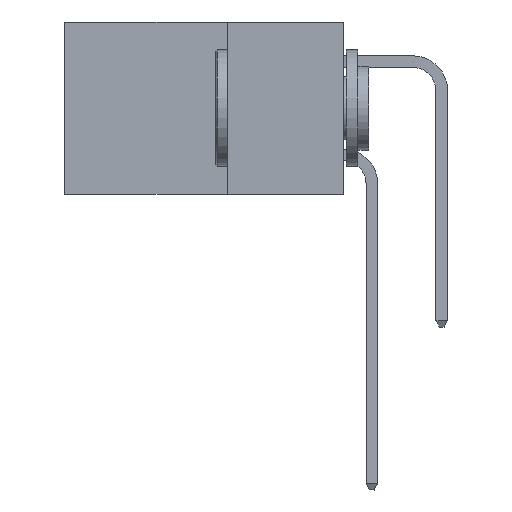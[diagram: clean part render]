
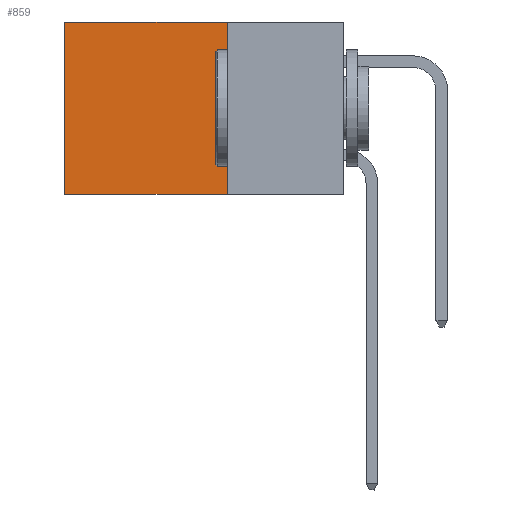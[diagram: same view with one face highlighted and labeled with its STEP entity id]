
A CAD part, left-side view. The second image highlights one B-rep face of the part: STEP entity #859.
In plain terms, the highlighted planar face has unit normal (-1, 0, 0).
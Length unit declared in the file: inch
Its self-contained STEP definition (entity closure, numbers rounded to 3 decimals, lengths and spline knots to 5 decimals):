
#859 = ADVANCED_FACE ( 'NONE', ( #1361 ), #1372, .F. ) ;
#956 = EDGE_CURVE ( 'NONE', #3235, #8880, #4372, .T. ) ;
#1049 = VECTOR ( 'NONE', #12435, 39.37008 ) ;
#1361 = FACE_OUTER_BOUND ( 'NONE', #3888, .T. ) ;
#1372 = PLANE ( 'NONE',  #4037 ) ;
#1467 = CARTESIAN_POINT ( 'NONE',  ( 0.298, 0.6, 0. ) ) ;
#2017 = VECTOR ( 'NONE', #2345, 39.37008 ) ;
#2297 = EDGE_CURVE ( 'NONE', #3453, #7307, #4333, .T. ) ;
#2336 = ORIENTED_EDGE ( 'NONE', *, *, #2297, .T. ) ;
#2345 = DIRECTION ( 'NONE',  ( 0., 1., 0. ) ) ;
#3235 = VERTEX_POINT ( 'NONE', #12936 ) ;
#3274 = DIRECTION ( 'NONE',  ( 0., 0., -1. ) ) ;
#3366 = DIRECTION ( 'NONE',  ( 1., 0., 0. ) ) ;
#3453 = VERTEX_POINT ( 'NONE', #1467 ) ;
#3822 = ORIENTED_EDGE ( 'NONE', *, *, #12918, .F. ) ;
#3888 = EDGE_LOOP ( 'NONE', ( #2336, #3822, #10814, #8629 ) ) ;
#4037 = AXIS2_PLACEMENT_3D ( 'NONE', #7252, #3366, #3274 ) ;
#4333 = LINE ( 'NONE', #12934, #6229 ) ;
#4372 = LINE ( 'NONE', #9491, #1049 ) ;
#4547 = CARTESIAN_POINT ( 'NONE',  ( 0.298, 0.25, 0. ) ) ;
#6229 = VECTOR ( 'NONE', #11731, 39.37008 ) ;
#6628 = DIRECTION ( 'NONE',  ( 0., 1., 0. ) ) ;
#7252 = CARTESIAN_POINT ( 'NONE',  ( 0.298, 0.25, 0. ) ) ;
#7307 = VERTEX_POINT ( 'NONE', #8774 ) ;
#8629 = ORIENTED_EDGE ( 'NONE', *, *, #12271, .T. ) ;
#8774 = CARTESIAN_POINT ( 'NONE',  ( 0.298, 0.6, -0.37 ) ) ;
#8880 = VERTEX_POINT ( 'NONE', #9596 ) ;
#9491 = CARTESIAN_POINT ( 'NONE',  ( 0.298, 0.25, 0. ) ) ;
#9596 = CARTESIAN_POINT ( 'NONE',  ( 0.298, 0.25, -0.37 ) ) ;
#10814 = ORIENTED_EDGE ( 'NONE', *, *, #956, .F. ) ;
#11626 = VECTOR ( 'NONE', #6628, 39.37008 ) ;
#11731 = DIRECTION ( 'NONE',  ( 0., 0., -1. ) ) ;
#12271 = EDGE_CURVE ( 'NONE', #3235, #3453, #13052, .T. ) ;
#12381 = LINE ( 'NONE', #12422, #2017 ) ;
#12422 = CARTESIAN_POINT ( 'NONE',  ( 0.298, 0.25, -0.37 ) ) ;
#12435 = DIRECTION ( 'NONE',  ( 0., 0., -1. ) ) ;
#12918 = EDGE_CURVE ( 'NONE', #8880, #7307, #12381, .T. ) ;
#12934 = CARTESIAN_POINT ( 'NONE',  ( 0.298, 0.6, 0. ) ) ;
#12936 = CARTESIAN_POINT ( 'NONE',  ( 0.298, 0.25, 0. ) ) ;
#13052 = LINE ( 'NONE', #4547, #11626 ) ;
